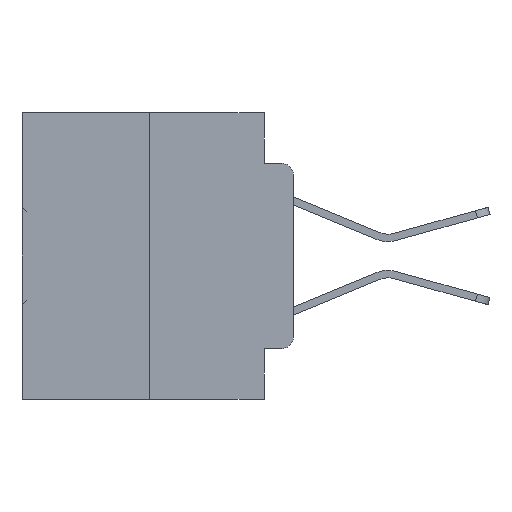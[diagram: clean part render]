
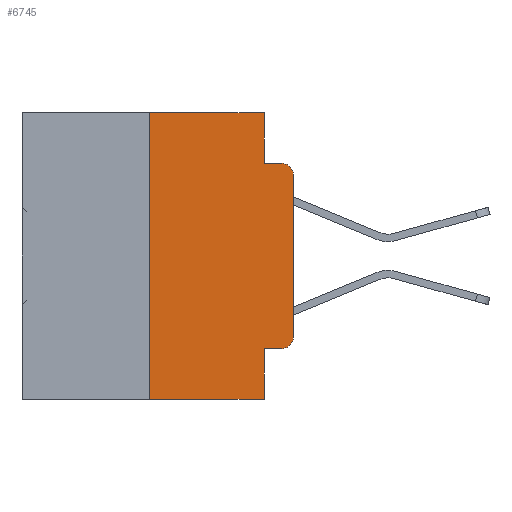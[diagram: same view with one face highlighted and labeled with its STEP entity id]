
A CAD part, left-side view. The second image highlights one B-rep face of the part: STEP entity #6745.
In plain terms, the highlighted planar face has unit normal (-1, 0, 0).
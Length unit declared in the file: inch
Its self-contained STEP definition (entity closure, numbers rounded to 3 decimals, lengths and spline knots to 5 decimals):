
#51 = EDGE_CURVE ( 'NONE', #23383, #14824, #8866, .T. ) ;
#261 = LINE ( 'NONE', #19588, #15915 ) ;
#977 = LINE ( 'NONE', #25818, #28872 ) ;
#1585 = CARTESIAN_POINT ( 'NONE',  ( 0., 0.051, -0.0885 ) ) ;
#1742 = ORIENTED_EDGE ( 'NONE', *, *, #25028, .F. ) ;
#1819 = DIRECTION ( 'NONE',  ( 0., 0., -1. ) ) ;
#2367 = CARTESIAN_POINT ( 'NONE',  ( 0., 0.02, -0.3915 ) ) ;
#2475 = EDGE_CURVE ( 'NONE', #9381, #21652, #977, .T. ) ;
#2850 = CARTESIAN_POINT ( 'NONE',  ( 0., 0., -0.3915 ) ) ;
#3044 = EDGE_CURVE ( 'NONE', #33888, #14824, #29681, .T. ) ;
#3530 = DIRECTION ( 'NONE',  ( 0., -1., 0. ) ) ;
#4198 = DIRECTION ( 'NONE',  ( 0., -1., 0. ) ) ;
#4408 = EDGE_CURVE ( 'NONE', #9381, #12082, #24844, .T. ) ;
#4415 = AXIS2_PLACEMENT_3D ( 'NONE', #27359, #25149, #29394 ) ;
#6408 = ORIENTED_EDGE ( 'NONE', *, *, #35494, .F. ) ;
#6424 = CARTESIAN_POINT ( 'NONE',  ( 0., 0.051, -0.5 ) ) ;
#6745 = ADVANCED_FACE ( 'NONE', ( #22664 ), #33917, .F. ) ;
#6933 = AXIS2_PLACEMENT_3D ( 'NONE', #2367, #36025, #1819 ) ;
#7121 = DIRECTION ( 'NONE',  ( 0., -1., 0. ) ) ;
#7306 = CARTESIAN_POINT ( 'NONE',  ( 0., 0.051, -0.4115 ) ) ;
#7479 = EDGE_CURVE ( 'NONE', #9880, #33139, #21029, .T. ) ;
#7510 = LINE ( 'NONE', #35477, #10346 ) ;
#7938 = EDGE_CURVE ( 'NONE', #33139, #33888, #14058, .T. ) ;
#8235 = CARTESIAN_POINT ( 'NONE',  ( 0., 0., -0.1085 ) ) ;
#8327 = CARTESIAN_POINT ( 'NONE',  ( 0., 0.473, -0.5 ) ) ;
#8866 = LINE ( 'NONE', #12396, #26161 ) ;
#9381 = VERTEX_POINT ( 'NONE', #11695 ) ;
#9880 = VERTEX_POINT ( 'NONE', #26687 ) ;
#10170 = ORIENTED_EDGE ( 'NONE', *, *, #16593, .F. ) ;
#10346 = VECTOR ( 'NONE', #4198, 39.37008 ) ;
#10637 = ORIENTED_EDGE ( 'NONE', *, *, #7938, .T. ) ;
#11695 = CARTESIAN_POINT ( 'NONE',  ( 0., 0.25, -0.5 ) ) ;
#11864 = DIRECTION ( 'NONE',  ( 0., 0., -1. ) ) ;
#12082 = VERTEX_POINT ( 'NONE', #6424 ) ;
#12396 = CARTESIAN_POINT ( 'NONE',  ( 0., 0.051, -0.0885 ) ) ;
#12470 = LINE ( 'NONE', #24036, #26163 ) ;
#12678 = VERTEX_POINT ( 'NONE', #7306 ) ;
#14058 = LINE ( 'NONE', #22138, #24576 ) ;
#14148 = LINE ( 'NONE', #22225, #25022 ) ;
#14824 = VERTEX_POINT ( 'NONE', #33687 ) ;
#15915 = VECTOR ( 'NONE', #11864, 39.37008 ) ;
#16593 = EDGE_CURVE ( 'NONE', #12678, #12082, #14148, .T. ) ;
#16804 = VECTOR ( 'NONE', #34349, 39.37008 ) ;
#18026 = AXIS2_PLACEMENT_3D ( 'NONE', #20264, #34093, #34639 ) ;
#18813 = ORIENTED_EDGE ( 'NONE', *, *, #4408, .T. ) ;
#19194 = DIRECTION ( 'NONE',  ( 0., 0., 1. ) ) ;
#19588 = CARTESIAN_POINT ( 'NONE',  ( 0., 0.051, 0. ) ) ;
#20264 = CARTESIAN_POINT ( 'NONE',  ( 0., 0.473, 0. ) ) ;
#21029 = CIRCLE ( 'NONE', #6933, 0.02 ) ;
#21652 = VERTEX_POINT ( 'NONE', #32150 ) ;
#22138 = CARTESIAN_POINT ( 'NONE',  ( 0., 0., 0. ) ) ;
#22225 = CARTESIAN_POINT ( 'NONE',  ( 0., 0.051, 0. ) ) ;
#22664 = FACE_OUTER_BOUND ( 'NONE', #35197, .T. ) ;
#23047 = DIRECTION ( 'NONE',  ( 0., 0., 1. ) ) ;
#23383 = VERTEX_POINT ( 'NONE', #1585 ) ;
#24036 = CARTESIAN_POINT ( 'NONE',  ( 0., 0.051, -0.4115 ) ) ;
#24506 = ORIENTED_EDGE ( 'NONE', *, *, #3044, .T. ) ;
#24576 = VECTOR ( 'NONE', #19194, 39.37008 ) ;
#24844 = LINE ( 'NONE', #8327, #16804 ) ;
#25022 = VECTOR ( 'NONE', #36030, 39.37008 ) ;
#25028 = EDGE_CURVE ( 'NONE', #27569, #23383, #261, .T. ) ;
#25149 = DIRECTION ( 'NONE',  ( -1., 0., 0. ) ) ;
#25818 = CARTESIAN_POINT ( 'NONE',  ( 0., 0.25, 0. ) ) ;
#26161 = VECTOR ( 'NONE', #3530, 39.37008 ) ;
#26163 = VECTOR ( 'NONE', #7121, 39.37008 ) ;
#26687 = CARTESIAN_POINT ( 'NONE',  ( 0., 0.02, -0.4115 ) ) ;
#27359 = CARTESIAN_POINT ( 'NONE',  ( 0., 0.02, -0.1085 ) ) ;
#27569 = VERTEX_POINT ( 'NONE', #30066 ) ;
#28872 = VECTOR ( 'NONE', #23047, 39.37008 ) ;
#29394 = DIRECTION ( 'NONE',  ( 0., 0., -1. ) ) ;
#29681 = CIRCLE ( 'NONE', #4415, 0.02 ) ;
#30066 = CARTESIAN_POINT ( 'NONE',  ( 0., 0.051, 0. ) ) ;
#30348 = ORIENTED_EDGE ( 'NONE', *, *, #51, .F. ) ;
#30782 = ORIENTED_EDGE ( 'NONE', *, *, #2475, .F. ) ;
#31244 = ORIENTED_EDGE ( 'NONE', *, *, #7479, .T. ) ;
#32150 = CARTESIAN_POINT ( 'NONE',  ( 0., 0.25, 0. ) ) ;
#32885 = EDGE_CURVE ( 'NONE', #12678, #9880, #12470, .T. ) ;
#33139 = VERTEX_POINT ( 'NONE', #2850 ) ;
#33687 = CARTESIAN_POINT ( 'NONE',  ( 0., 0.02, -0.0885 ) ) ;
#33888 = VERTEX_POINT ( 'NONE', #8235 ) ;
#33917 = PLANE ( 'NONE',  #18026 ) ;
#34093 = DIRECTION ( 'NONE',  ( 1., 0., 0. ) ) ;
#34349 = DIRECTION ( 'NONE',  ( 0., -1., 0. ) ) ;
#34639 = DIRECTION ( 'NONE',  ( 0., 0., -1. ) ) ;
#35197 = EDGE_LOOP ( 'NONE', ( #10637, #24506, #30348, #1742, #6408, #30782, #18813, #10170, #35793, #31244 ) ) ;
#35477 = CARTESIAN_POINT ( 'NONE',  ( 0., 0.473, 0. ) ) ;
#35494 = EDGE_CURVE ( 'NONE', #21652, #27569, #7510, .T. ) ;
#35793 = ORIENTED_EDGE ( 'NONE', *, *, #32885, .T. ) ;
#36025 = DIRECTION ( 'NONE',  ( -1., 0., 0. ) ) ;
#36030 = DIRECTION ( 'NONE',  ( 0., 0., -1. ) ) ;
